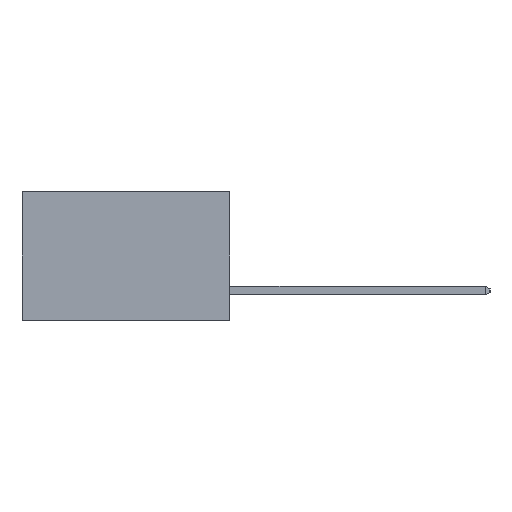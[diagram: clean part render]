
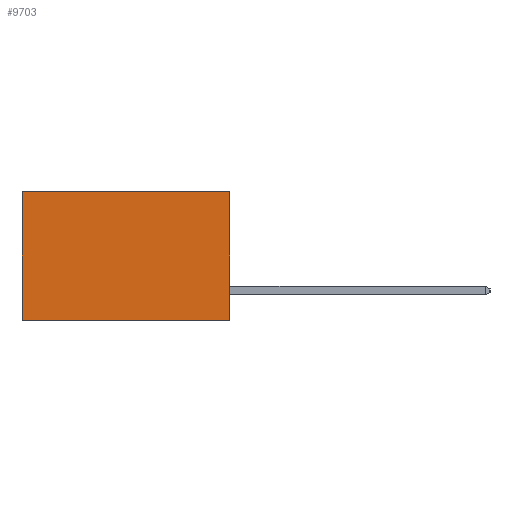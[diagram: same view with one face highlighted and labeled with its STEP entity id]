
A CAD part, left-side view. The second image highlights one B-rep face of the part: STEP entity #9703.
In plain terms, the highlighted planar face has unit normal (-1, 0, 0).
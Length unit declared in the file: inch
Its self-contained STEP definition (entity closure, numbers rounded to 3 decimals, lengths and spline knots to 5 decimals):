
#363 = DIRECTION ( 'NONE',  ( 0., 1., 0. ) ) ;
#391 = CARTESIAN_POINT ( 'NONE',  ( 0.298, 0., 0. ) ) ;
#866 = VECTOR ( 'NONE', #363, 39.37008 ) ;
#1510 = EDGE_LOOP ( 'NONE', ( #5338, #1989, #19652, #13828 ) ) ;
#1671 = VECTOR ( 'NONE', #10907, 39.37008 ) ;
#1809 = DIRECTION ( 'NONE',  ( 0., 0., -1. ) ) ;
#1989 = ORIENTED_EDGE ( 'NONE', *, *, #11405, .F. ) ;
#2065 = EDGE_CURVE ( 'NONE', #8687, #16120, #2218, .T. ) ;
#2218 = LINE ( 'NONE', #10973, #1671 ) ;
#2944 = FACE_OUTER_BOUND ( 'NONE', #1510, .T. ) ;
#3842 = VERTEX_POINT ( 'NONE', #6620 ) ;
#3889 = PLANE ( 'NONE',  #8816 ) ;
#4760 = EDGE_CURVE ( 'NONE', #8687, #6018, #5026, .T. ) ;
#4990 = CARTESIAN_POINT ( 'NONE',  ( 0.298, 0.6, 0. ) ) ;
#5026 = LINE ( 'NONE', #391, #866 ) ;
#5338 = ORIENTED_EDGE ( 'NONE', *, *, #8970, .T. ) ;
#6018 = VERTEX_POINT ( 'NONE', #15277 ) ;
#6620 = CARTESIAN_POINT ( 'NONE',  ( 0.298, 0.6, -0.37 ) ) ;
#7582 = VECTOR ( 'NONE', #15703, 39.37008 ) ;
#8180 = LINE ( 'NONE', #4990, #16342 ) ;
#8687 = VERTEX_POINT ( 'NONE', #15351 ) ;
#8816 = AXIS2_PLACEMENT_3D ( 'NONE', #15427, #20633, #20582 ) ;
#8970 = EDGE_CURVE ( 'NONE', #6018, #3842, #8180, .T. ) ;
#9703 = ADVANCED_FACE ( 'NONE', ( #2944 ), #3889, .F. ) ;
#10907 = DIRECTION ( 'NONE',  ( 0., 0., -1. ) ) ;
#10973 = CARTESIAN_POINT ( 'NONE',  ( 0.298, 0., 0. ) ) ;
#11405 = EDGE_CURVE ( 'NONE', #16120, #3842, #16263, .T. ) ;
#13828 = ORIENTED_EDGE ( 'NONE', *, *, #4760, .T. ) ;
#14754 = CARTESIAN_POINT ( 'NONE',  ( 0.298, 0., -0.37 ) ) ;
#15277 = CARTESIAN_POINT ( 'NONE',  ( 0.298, 0.6, 0. ) ) ;
#15351 = CARTESIAN_POINT ( 'NONE',  ( 0.298, 0., 0. ) ) ;
#15427 = CARTESIAN_POINT ( 'NONE',  ( 0.298, 0., 0. ) ) ;
#15703 = DIRECTION ( 'NONE',  ( 0., 1., 0. ) ) ;
#15725 = CARTESIAN_POINT ( 'NONE',  ( 0.298, 0., -0.37 ) ) ;
#16120 = VERTEX_POINT ( 'NONE', #14754 ) ;
#16263 = LINE ( 'NONE', #15725, #7582 ) ;
#16342 = VECTOR ( 'NONE', #1809, 39.37008 ) ;
#19652 = ORIENTED_EDGE ( 'NONE', *, *, #2065, .F. ) ;
#20582 = DIRECTION ( 'NONE',  ( 0., 0., -1. ) ) ;
#20633 = DIRECTION ( 'NONE',  ( 1., 0., 0. ) ) ;
